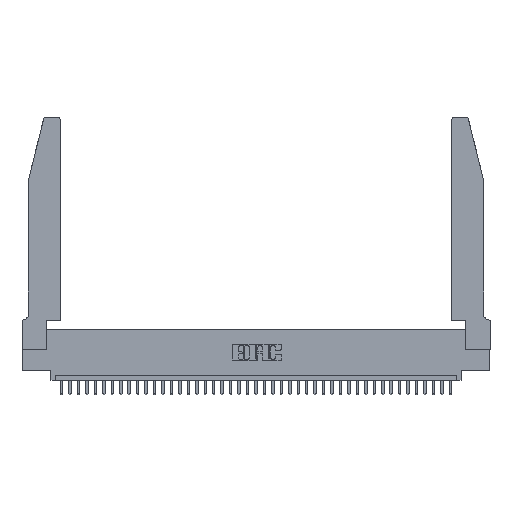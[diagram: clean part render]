
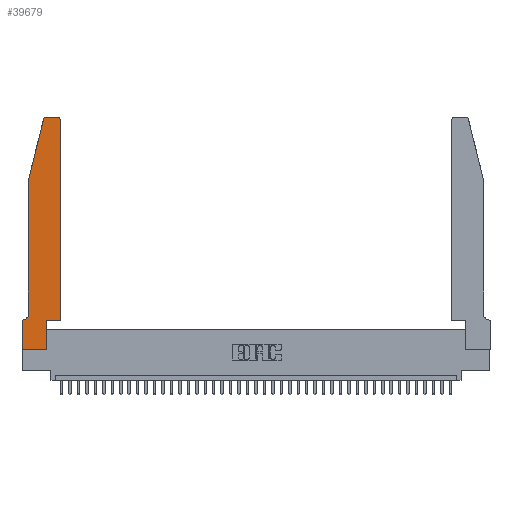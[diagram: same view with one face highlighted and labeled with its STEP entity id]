
A CAD part, top view. The second image highlights one B-rep face of the part: STEP entity #39679.
In plain terms, the highlighted planar face has unit normal (0, 0, 1).
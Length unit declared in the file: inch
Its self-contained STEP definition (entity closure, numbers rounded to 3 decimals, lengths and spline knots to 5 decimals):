
#1200 = VERTEX_POINT ( 'NONE', #19151 ) ;
#1497 = ORIENTED_EDGE ( 'NONE', *, *, #4478, .T. ) ;
#2235 = CARTESIAN_POINT ( 'NONE',  ( 0.0755, 0.42, 0.37 ) ) ;
#2243 = CARTESIAN_POINT ( 'NONE',  ( 0.4205, 2.75, 0.37 ) ) ;
#2257 = CARTESIAN_POINT ( 'NONE',  ( 0.4505, 0.35, 0.37 ) ) ;
#2259 = LINE ( 'NONE', #2257, #21441 ) ;
#2435 = CARTESIAN_POINT ( 'NONE',  ( 0.0755, 2., 0.37 ) ) ;
#2505 = EDGE_CURVE ( 'NONE', #4710, #6268, #2259, .T. ) ;
#2510 = EDGE_CURVE ( 'NONE', #21031, #29162, #6095, .T. ) ;
#3617 = AXIS2_PLACEMENT_3D ( 'NONE', #36456, #24476, #18564 ) ;
#3952 = ORIENTED_EDGE ( 'NONE', *, *, #27397, .T. ) ;
#4020 = CIRCLE ( 'NONE', #12854, 0.07 ) ;
#4478 = EDGE_CURVE ( 'NONE', #21442, #21031, #5022, .T. ) ;
#4710 = VERTEX_POINT ( 'NONE', #16630 ) ;
#4891 = DIRECTION ( 'NONE',  ( 0., 0., 1. ) ) ;
#4958 = ORIENTED_EDGE ( 'NONE', *, *, #19839, .T. ) ;
#5022 = CIRCLE ( 'NONE', #19953, 0.03 ) ;
#6095 = LINE ( 'NONE', #35765, #18522 ) ;
#6268 = VERTEX_POINT ( 'NONE', #29887 ) ;
#6331 = VECTOR ( 'NONE', #26759, 39.37008 ) ;
#6351 = VERTEX_POINT ( 'NONE', #2243 ) ;
#6465 = EDGE_CURVE ( 'NONE', #23755, #35957, #29228, .T. ) ;
#7178 = CARTESIAN_POINT ( 'NONE',  ( 0., 0., 0.37 ) ) ;
#7353 = VECTOR ( 'NONE', #22728, 39.37008 ) ;
#7673 = CARTESIAN_POINT ( 'NONE',  ( 0.2865, 0.35, 0.37 ) ) ;
#7936 = DIRECTION ( 'NONE',  ( 0., 1., 0. ) ) ;
#8690 = DIRECTION ( 'NONE',  ( 1., 0., 0. ) ) ;
#9690 = ORIENTED_EDGE ( 'NONE', *, *, #14305, .T. ) ;
#10144 = VERTEX_POINT ( 'NONE', #37936 ) ;
#11524 = CARTESIAN_POINT ( 'NONE',  ( 0., 0., 0.37 ) ) ;
#11989 = EDGE_CURVE ( 'NONE', #35957, #10144, #21418, .T. ) ;
#12511 = FACE_OUTER_BOUND ( 'NONE', #32740, .T. ) ;
#12854 = AXIS2_PLACEMENT_3D ( 'NONE', #34513, #18942, #31245 ) ;
#12877 = ORIENTED_EDGE ( 'NONE', *, *, #6465, .T. ) ;
#13686 = VECTOR ( 'NONE', #35945, 39.37008 ) ;
#14305 = EDGE_CURVE ( 'NONE', #21349, #23755, #19240, .T. ) ;
#14393 = EDGE_CURVE ( 'NONE', #6351, #21442, #18275, .T. ) ;
#14523 = CIRCLE ( 'NONE', #30599, 0.03 ) ;
#14873 = DIRECTION ( 'NONE',  ( -1., 0., 0. ) ) ;
#15841 = CARTESIAN_POINT ( 'NONE',  ( 0.25487, 2.72718, 0.37 ) ) ;
#15947 = EDGE_CURVE ( 'NONE', #10144, #4710, #22961, .T. ) ;
#16630 = CARTESIAN_POINT ( 'NONE',  ( 0.2865, 0.35, 0.37 ) ) ;
#16836 = ORIENTED_EDGE ( 'NONE', *, *, #18975, .T. ) ;
#17970 = DIRECTION ( 'NONE',  ( -1., 0., 0. ) ) ;
#18275 = LINE ( 'NONE', #27872, #25947 ) ;
#18522 = VECTOR ( 'NONE', #35629, 39.37008 ) ;
#18564 = DIRECTION ( 'NONE',  ( 1., 0., 0. ) ) ;
#18942 = DIRECTION ( 'NONE',  ( 0., 0., -1. ) ) ;
#18975 = EDGE_CURVE ( 'NONE', #20967, #21349, #4020, .T. ) ;
#19151 = CARTESIAN_POINT ( 'NONE',  ( 0.4505, 2.72, 0.37 ) ) ;
#19240 = LINE ( 'NONE', #37706, #20737 ) ;
#19522 = CARTESIAN_POINT ( 'NONE',  ( 0.0055, 0.35, 0.37 ) ) ;
#19734 = LINE ( 'NONE', #35914, #6331 ) ;
#19839 = EDGE_CURVE ( 'NONE', #1200, #6351, #14523, .T. ) ;
#19953 = AXIS2_PLACEMENT_3D ( 'NONE', #38540, #4891, #29217 ) ;
#20381 = DIRECTION ( 'NONE',  ( 0., -1., 0. ) ) ;
#20606 = DIRECTION ( 'NONE',  ( 0., 0., 1. ) ) ;
#20737 = VECTOR ( 'NONE', #14873, 39.37008 ) ;
#20806 = LINE ( 'NONE', #27812, #7353 ) ;
#20967 = VERTEX_POINT ( 'NONE', #2235 ) ;
#21031 = VERTEX_POINT ( 'NONE', #15841 ) ;
#21349 = VERTEX_POINT ( 'NONE', #19522 ) ;
#21418 = LINE ( 'NONE', #29717, #13686 ) ;
#21441 = VECTOR ( 'NONE', #8690, 39.37008 ) ;
#21442 = VERTEX_POINT ( 'NONE', #26348 ) ;
#21991 = VECTOR ( 'NONE', #7936, 39.37008 ) ;
#22728 = DIRECTION ( 'NONE',  ( 0., -1., 0. ) ) ;
#22961 = LINE ( 'NONE', #7673, #21991 ) ;
#23024 = ORIENTED_EDGE ( 'NONE', *, *, #39514, .T. ) ;
#23394 = CARTESIAN_POINT ( 'NONE',  ( 0.4205, 2.72, 0.37 ) ) ;
#23755 = VERTEX_POINT ( 'NONE', #36128 ) ;
#23795 = DIRECTION ( 'NONE',  ( 1., 0., 0. ) ) ;
#24476 = DIRECTION ( 'NONE',  ( 0., 0., 1. ) ) ;
#25947 = VECTOR ( 'NONE', #17970, 39.37008 ) ;
#26348 = CARTESIAN_POINT ( 'NONE',  ( 0.284, 2.75, 0.37 ) ) ;
#26759 = DIRECTION ( 'NONE',  ( 0., 1., 0. ) ) ;
#27397 = EDGE_CURVE ( 'NONE', #29162, #20967, #20806, .T. ) ;
#27812 = CARTESIAN_POINT ( 'NONE',  ( 0.0755, 2., 0.37 ) ) ;
#27872 = CARTESIAN_POINT ( 'NONE',  ( 0.2605, 2.75, 0.37 ) ) ;
#27935 = ORIENTED_EDGE ( 'NONE', *, *, #2510, .T. ) ;
#29162 = VERTEX_POINT ( 'NONE', #2435 ) ;
#29217 = DIRECTION ( 'NONE',  ( 1., 0., 0. ) ) ;
#29228 = LINE ( 'NONE', #11524, #35055 ) ;
#29717 = CARTESIAN_POINT ( 'NONE',  ( 0., 0., 0.37 ) ) ;
#29887 = CARTESIAN_POINT ( 'NONE',  ( 0.4505, 0.35, 0.37 ) ) ;
#30599 = AXIS2_PLACEMENT_3D ( 'NONE', #23394, #20606, #23795 ) ;
#31245 = DIRECTION ( 'NONE',  ( -1., 0., 0. ) ) ;
#32583 = ORIENTED_EDGE ( 'NONE', *, *, #15947, .T. ) ;
#32740 = EDGE_LOOP ( 'NONE', ( #36308, #1497, #27935, #3952, #16836, #9690, #12877, #34792, #32583, #34941, #23024, #4958 ) ) ;
#33363 = PLANE ( 'NONE',  #3617 ) ;
#34513 = CARTESIAN_POINT ( 'NONE',  ( 0.0055, 0.42, 0.37 ) ) ;
#34792 = ORIENTED_EDGE ( 'NONE', *, *, #11989, .T. ) ;
#34941 = ORIENTED_EDGE ( 'NONE', *, *, #2505, .T. ) ;
#35055 = VECTOR ( 'NONE', #20381, 39.37008 ) ;
#35629 = DIRECTION ( 'NONE',  ( -0.239, -0.971, 0. ) ) ;
#35765 = CARTESIAN_POINT ( 'NONE',  ( 0.0755, 2., 0.37 ) ) ;
#35914 = CARTESIAN_POINT ( 'NONE',  ( 0.4505, 0.35, 0.37 ) ) ;
#35945 = DIRECTION ( 'NONE',  ( 1., 0., 0. ) ) ;
#35957 = VERTEX_POINT ( 'NONE', #7178 ) ;
#36128 = CARTESIAN_POINT ( 'NONE',  ( 0., 0.35, 0.37 ) ) ;
#36308 = ORIENTED_EDGE ( 'NONE', *, *, #14393, .T. ) ;
#36456 = CARTESIAN_POINT ( 'NONE',  ( 0., 0.35, 0.37 ) ) ;
#37706 = CARTESIAN_POINT ( 'NONE',  ( 0.0755, 0.35, 0.37 ) ) ;
#37936 = CARTESIAN_POINT ( 'NONE',  ( 0.2865, 0., 0.37 ) ) ;
#38540 = CARTESIAN_POINT ( 'NONE',  ( 0.284, 2.72, 0.37 ) ) ;
#39514 = EDGE_CURVE ( 'NONE', #6268, #1200, #19734, .T. ) ;
#39679 = ADVANCED_FACE ( 'NONE', ( #12511 ), #33363, .T. ) ;
